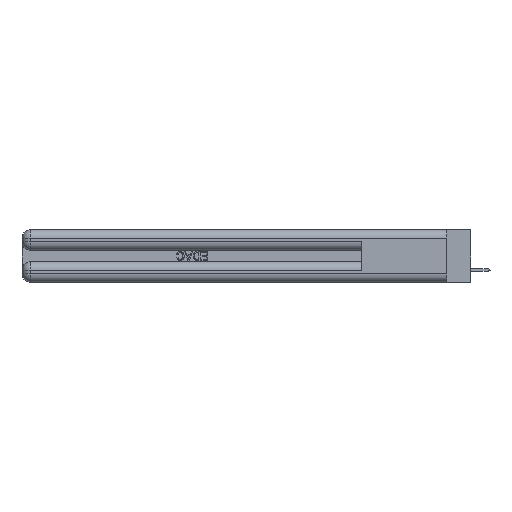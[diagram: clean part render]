
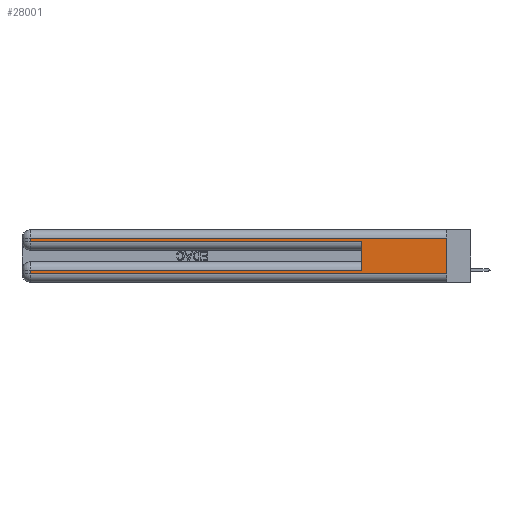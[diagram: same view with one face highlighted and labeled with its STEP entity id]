
A CAD part, left-side view. The second image highlights one B-rep face of the part: STEP entity #28001.
In plain terms, the highlighted planar face has unit normal (-1, 0, 0).
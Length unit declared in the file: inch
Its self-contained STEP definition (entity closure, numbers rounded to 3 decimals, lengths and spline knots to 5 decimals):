
#1165 = CARTESIAN_POINT ( 'NONE',  ( 0., 2.94, 0.06 ) ) ;
#1347 = LINE ( 'NONE', #8860, #35701 ) ;
#2022 = VECTOR ( 'NONE', #4412, 39.37008 ) ;
#2331 = ORIENTED_EDGE ( 'NONE', *, *, #39860, .F. ) ;
#2682 = VERTEX_POINT ( 'NONE', #40650 ) ;
#2812 = VERTEX_POINT ( 'NONE', #31064 ) ;
#3283 = EDGE_CURVE ( 'NONE', #41260, #30093, #17705, .T. ) ;
#3291 = ORIENTED_EDGE ( 'NONE', *, *, #37245, .T. ) ;
#3951 = DIRECTION ( 'NONE',  ( 0., 0., -1. ) ) ;
#4412 = DIRECTION ( 'NONE',  ( 0., 1., 0. ) ) ;
#4594 = CARTESIAN_POINT ( 'NONE',  ( 0., 0.6, 0.285 ) ) ;
#4799 = CARTESIAN_POINT ( 'NONE',  ( 0., 2.94, 0.085 ) ) ;
#5372 = CARTESIAN_POINT ( 'NONE',  ( 0., 2.94, 0.37 ) ) ;
#5374 = CARTESIAN_POINT ( 'NONE',  ( 0., 0.6, 0.085 ) ) ;
#6706 = EDGE_LOOP ( 'NONE', ( #2331, #30495, #37826, #38685, #27749, #28948, #10873, #3291 ) ) ;
#7001 = VERTEX_POINT ( 'NONE', #8888 ) ;
#7370 = PLANE ( 'NONE',  #28837 ) ;
#8813 = LINE ( 'NONE', #36633, #30674 ) ;
#8860 = CARTESIAN_POINT ( 'NONE',  ( 0., 0., 0.31 ) ) ;
#8888 = CARTESIAN_POINT ( 'NONE',  ( 0., 2.94, 0.285 ) ) ;
#10329 = VECTOR ( 'NONE', #23058, 39.37008 ) ;
#10873 = ORIENTED_EDGE ( 'NONE', *, *, #3283, .T. ) ;
#12661 = DIRECTION ( 'NONE',  ( 0., 0., -1. ) ) ;
#13616 = VECTOR ( 'NONE', #22472, 39.37008 ) ;
#15117 = CARTESIAN_POINT ( 'NONE',  ( 0., 0., 0.085 ) ) ;
#15619 = CARTESIAN_POINT ( 'NONE',  ( 0., 2.94, 0.37 ) ) ;
#16200 = LINE ( 'NONE', #23286, #10329 ) ;
#16429 = LINE ( 'NONE', #33100, #27131 ) ;
#17705 = LINE ( 'NONE', #15619, #13616 ) ;
#18201 = EDGE_CURVE ( 'NONE', #2812, #37683, #1347, .T. ) ;
#18259 = CARTESIAN_POINT ( 'NONE',  ( 0., 2.94, 0.31 ) ) ;
#20769 = EDGE_CURVE ( 'NONE', #34424, #38890, #16429, .T. ) ;
#21285 = CARTESIAN_POINT ( 'NONE',  ( 0., 0., 0.37 ) ) ;
#21567 = EDGE_CURVE ( 'NONE', #7001, #38890, #16200, .T. ) ;
#21751 = LINE ( 'NONE', #15117, #2022 ) ;
#21963 = CARTESIAN_POINT ( 'NONE',  ( 0., 0., 0.06 ) ) ;
#22472 = DIRECTION ( 'NONE',  ( 0., 0., -1. ) ) ;
#23058 = DIRECTION ( 'NONE',  ( 0., -1., 0. ) ) ;
#23286 = CARTESIAN_POINT ( 'NONE',  ( 0., 0., 0.285 ) ) ;
#25502 = DIRECTION ( 'NONE',  ( 0., 1., 0. ) ) ;
#26710 = DIRECTION ( 'NONE',  ( 0., 0., 1. ) ) ;
#27131 = VECTOR ( 'NONE', #26710, 39.37008 ) ;
#27749 = ORIENTED_EDGE ( 'NONE', *, *, #20769, .F. ) ;
#28001 = ADVANCED_FACE ( 'NONE', ( #34966 ), #7370, .F. ) ;
#28837 = AXIS2_PLACEMENT_3D ( 'NONE', #21285, #35190, #3951 ) ;
#28948 = ORIENTED_EDGE ( 'NONE', *, *, #31565, .T. ) ;
#29952 = LINE ( 'NONE', #21963, #43038 ) ;
#30093 = VERTEX_POINT ( 'NONE', #1165 ) ;
#30495 = ORIENTED_EDGE ( 'NONE', *, *, #18201, .T. ) ;
#30674 = VECTOR ( 'NONE', #37086, 39.37008 ) ;
#31064 = CARTESIAN_POINT ( 'NONE',  ( 0., 0., 0.31 ) ) ;
#31565 = EDGE_CURVE ( 'NONE', #34424, #41260, #21751, .T. ) ;
#33100 = CARTESIAN_POINT ( 'NONE',  ( 0., 0.6, 0.145 ) ) ;
#34424 = VERTEX_POINT ( 'NONE', #5374 ) ;
#34966 = FACE_OUTER_BOUND ( 'NONE', #6706, .T. ) ;
#35120 = VECTOR ( 'NONE', #12661, 39.37008 ) ;
#35190 = DIRECTION ( 'NONE',  ( 1., 0., 0. ) ) ;
#35701 = VECTOR ( 'NONE', #25502, 39.37008 ) ;
#35880 = DIRECTION ( 'NONE',  ( 0., -1., 0. ) ) ;
#36633 = CARTESIAN_POINT ( 'NONE',  ( 0., 0., 0.37 ) ) ;
#36851 = EDGE_CURVE ( 'NONE', #37683, #7001, #43218, .T. ) ;
#37086 = DIRECTION ( 'NONE',  ( 0., 0., -1. ) ) ;
#37245 = EDGE_CURVE ( 'NONE', #30093, #2682, #29952, .T. ) ;
#37683 = VERTEX_POINT ( 'NONE', #18259 ) ;
#37826 = ORIENTED_EDGE ( 'NONE', *, *, #36851, .T. ) ;
#38685 = ORIENTED_EDGE ( 'NONE', *, *, #21567, .T. ) ;
#38890 = VERTEX_POINT ( 'NONE', #4594 ) ;
#39860 = EDGE_CURVE ( 'NONE', #2812, #2682, #8813, .T. ) ;
#40650 = CARTESIAN_POINT ( 'NONE',  ( 0., 0., 0.06 ) ) ;
#41260 = VERTEX_POINT ( 'NONE', #4799 ) ;
#43038 = VECTOR ( 'NONE', #35880, 39.37008 ) ;
#43218 = LINE ( 'NONE', #5372, #35120 ) ;
